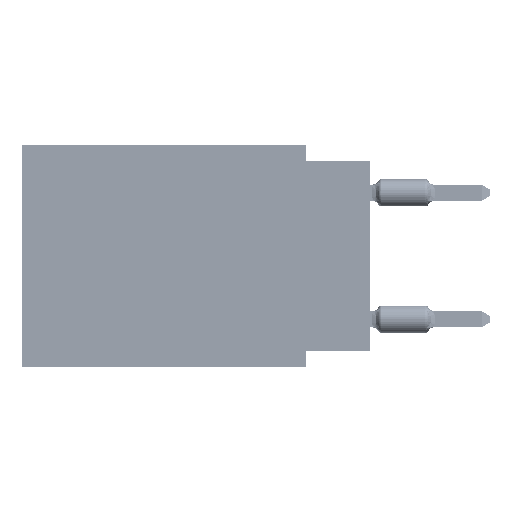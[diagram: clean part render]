
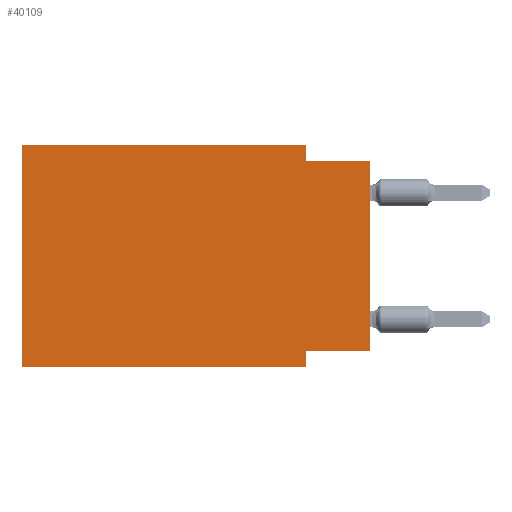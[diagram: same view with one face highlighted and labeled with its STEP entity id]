
A CAD part, left-side view. The second image highlights one B-rep face of the part: STEP entity #40109.
In plain terms, the highlighted planar face has unit normal (-1, 0, 0).
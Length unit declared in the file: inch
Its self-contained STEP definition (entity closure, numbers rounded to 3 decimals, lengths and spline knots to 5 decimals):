
#2501 = CARTESIAN_POINT ( 'NONE',  ( 0., 0.1, -0.025 ) ) ;
#3801 = AXIS2_PLACEMENT_3D ( 'NONE', #42424, #29780, #62032 ) ;
#4115 = VECTOR ( 'NONE', #72555, 39.37008 ) ;
#4650 = CARTESIAN_POINT ( 'NONE',  ( 0., 0., -0.325 ) ) ;
#5200 = ORIENTED_EDGE ( 'NONE', *, *, #14588, .F. ) ;
#7021 = VERTEX_POINT ( 'NONE', #74826 ) ;
#7178 = EDGE_CURVE ( 'NONE', #84346, #68625, #45994, .T. ) ;
#7745 = ORIENTED_EDGE ( 'NONE', *, *, #17506, .F. ) ;
#8059 = LINE ( 'NONE', #16617, #41199 ) ;
#11624 = DIRECTION ( 'NONE',  ( 0., 1., 0. ) ) ;
#13381 = CARTESIAN_POINT ( 'NONE',  ( 0., 0., -0.325 ) ) ;
#13838 = DIRECTION ( 'NONE',  ( 0., 0., 1. ) ) ;
#14494 = VECTOR ( 'NONE', #74038, 39.37008 ) ;
#14588 = EDGE_CURVE ( 'NONE', #58354, #7021, #43882, .T. ) ;
#15005 = ORIENTED_EDGE ( 'NONE', *, *, #82153, .T. ) ;
#15342 = CARTESIAN_POINT ( 'NONE',  ( 0., 0., -0.025 ) ) ;
#16617 = CARTESIAN_POINT ( 'NONE',  ( 0., 0.1, -0.35 ) ) ;
#16715 = DIRECTION ( 'NONE',  ( 0., 0., 1. ) ) ;
#17506 = EDGE_CURVE ( 'NONE', #29768, #84346, #75574, .T. ) ;
#17850 = VERTEX_POINT ( 'NONE', #15342 ) ;
#18111 = CARTESIAN_POINT ( 'NONE',  ( 0., 0.55, 0. ) ) ;
#18803 = VECTOR ( 'NONE', #30768, 39.37008 ) ;
#19169 = EDGE_CURVE ( 'NONE', #7021, #53656, #8059, .T. ) ;
#20129 = DIRECTION ( 'NONE',  ( 0., -1., 0. ) ) ;
#21699 = ORIENTED_EDGE ( 'NONE', *, *, #57534, .F. ) ;
#23081 = CARTESIAN_POINT ( 'NONE',  ( 0., 0.1, -0.35 ) ) ;
#23597 = CARTESIAN_POINT ( 'NONE',  ( 0., 0.55, -0.35 ) ) ;
#26575 = CARTESIAN_POINT ( 'NONE',  ( 0., 0.1, 0. ) ) ;
#26902 = ORIENTED_EDGE ( 'NONE', *, *, #66291, .F. ) ;
#27966 = LINE ( 'NONE', #34931, #79788 ) ;
#29768 = VERTEX_POINT ( 'NONE', #23597 ) ;
#29780 = DIRECTION ( 'NONE',  ( 1., 0., 0. ) ) ;
#30768 = DIRECTION ( 'NONE',  ( 0., -1., 0. ) ) ;
#33538 = LINE ( 'NONE', #26575, #14494 ) ;
#34931 = CARTESIAN_POINT ( 'NONE',  ( 0., 0., -0.025 ) ) ;
#36242 = EDGE_LOOP ( 'NONE', ( #15005, #21699, #26902, #51708, #7745, #42815, #78752, #5200 ) ) ;
#36331 = CARTESIAN_POINT ( 'NONE',  ( 0., 0.55, 0. ) ) ;
#36435 = CARTESIAN_POINT ( 'NONE',  ( 0., 0.55, -0.35 ) ) ;
#38850 = CARTESIAN_POINT ( 'NONE',  ( 0., 0.55, 0. ) ) ;
#40109 = ADVANCED_FACE ( 'NONE', ( #70273 ), #75531, .F. ) ;
#41199 = VECTOR ( 'NONE', #43212, 39.37008 ) ;
#42424 = CARTESIAN_POINT ( 'NONE',  ( 0., 0.55, 0. ) ) ;
#42815 = ORIENTED_EDGE ( 'NONE', *, *, #61664, .T. ) ;
#43212 = DIRECTION ( 'NONE',  ( 0., 0., -1. ) ) ;
#43882 = LINE ( 'NONE', #4650, #81162 ) ;
#45994 = LINE ( 'NONE', #18111, #4115 ) ;
#51708 = ORIENTED_EDGE ( 'NONE', *, *, #7178, .F. ) ;
#53656 = VERTEX_POINT ( 'NONE', #23081 ) ;
#57534 = EDGE_CURVE ( 'NONE', #68531, #17850, #27966, .T. ) ;
#58354 = VERTEX_POINT ( 'NONE', #13381 ) ;
#61664 = EDGE_CURVE ( 'NONE', #29768, #53656, #64306, .T. ) ;
#62032 = DIRECTION ( 'NONE',  ( 0., 0., -1. ) ) ;
#64306 = LINE ( 'NONE', #36435, #18803 ) ;
#64663 = VECTOR ( 'NONE', #16715, 39.37008 ) ;
#66291 = EDGE_CURVE ( 'NONE', #68625, #68531, #33538, .T. ) ;
#66562 = LINE ( 'NONE', #73100, #74898 ) ;
#68531 = VERTEX_POINT ( 'NONE', #2501 ) ;
#68625 = VERTEX_POINT ( 'NONE', #70466 ) ;
#70273 = FACE_OUTER_BOUND ( 'NONE', #36242, .T. ) ;
#70466 = CARTESIAN_POINT ( 'NONE',  ( 0., 0.1, 0. ) ) ;
#72555 = DIRECTION ( 'NONE',  ( 0., -1., 0. ) ) ;
#73100 = CARTESIAN_POINT ( 'NONE',  ( 0., 0., 0. ) ) ;
#74038 = DIRECTION ( 'NONE',  ( 0., 0., -1. ) ) ;
#74826 = CARTESIAN_POINT ( 'NONE',  ( 0., 0.1, -0.325 ) ) ;
#74898 = VECTOR ( 'NONE', #13838, 39.37008 ) ;
#75531 = PLANE ( 'NONE',  #3801 ) ;
#75574 = LINE ( 'NONE', #36331, #64663 ) ;
#78752 = ORIENTED_EDGE ( 'NONE', *, *, #19169, .F. ) ;
#79788 = VECTOR ( 'NONE', #20129, 39.37008 ) ;
#81162 = VECTOR ( 'NONE', #11624, 39.37008 ) ;
#82153 = EDGE_CURVE ( 'NONE', #58354, #17850, #66562, .T. ) ;
#84346 = VERTEX_POINT ( 'NONE', #38850 ) ;
